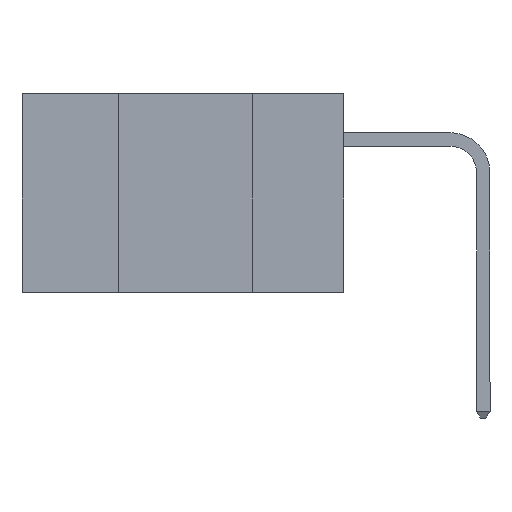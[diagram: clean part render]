
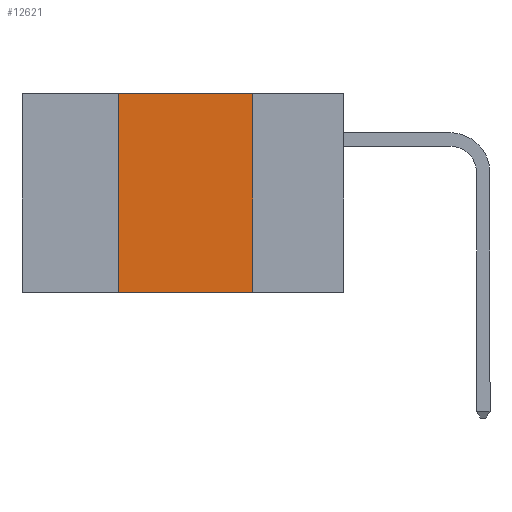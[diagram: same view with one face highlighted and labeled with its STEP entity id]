
A CAD part, left-side view. The second image highlights one B-rep face of the part: STEP entity #12621.
In plain terms, the highlighted planar face has unit normal (-1, 0, 0).
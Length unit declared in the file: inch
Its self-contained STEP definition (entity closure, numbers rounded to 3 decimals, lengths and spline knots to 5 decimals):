
#133 = DIRECTION ( 'NONE',  ( 0., 0., 1. ) ) ;
#1426 = EDGE_CURVE ( 'NONE', #14777, #12174, #7375, .T. ) ;
#1571 = CARTESIAN_POINT ( 'NONE',  ( 0., 0.42, -0.37 ) ) ;
#2990 = VERTEX_POINT ( 'NONE', #11616 ) ;
#3334 = EDGE_CURVE ( 'NONE', #15657, #2990, #10416, .T. ) ;
#4120 = EDGE_LOOP ( 'NONE', ( #12511, #9905, #12928, #5081 ) ) ;
#4126 = VECTOR ( 'NONE', #10595, 39.37008 ) ;
#4680 = DIRECTION ( 'NONE',  ( 0., -1., 0. ) ) ;
#5081 = ORIENTED_EDGE ( 'NONE', *, *, #3334, .T. ) ;
#6603 = VECTOR ( 'NONE', #4680, 39.37008 ) ;
#7154 = VECTOR ( 'NONE', #133, 39.37008 ) ;
#7375 = LINE ( 'NONE', #16394, #17864 ) ;
#7594 = LINE ( 'NONE', #14381, #7154 ) ;
#8070 = PLANE ( 'NONE',  #17657 ) ;
#9606 = DIRECTION ( 'NONE',  ( 0., 0., -1. ) ) ;
#9704 = EDGE_CURVE ( 'NONE', #15657, #14777, #7594, .T. ) ;
#9905 = ORIENTED_EDGE ( 'NONE', *, *, #1426, .F. ) ;
#10416 = LINE ( 'NONE', #12460, #6603 ) ;
#10595 = DIRECTION ( 'NONE',  ( 0., 0., -1. ) ) ;
#11380 = CARTESIAN_POINT ( 'NONE',  ( 0., 0.17, 0. ) ) ;
#11616 = CARTESIAN_POINT ( 'NONE',  ( 0., 0.17, -0.37 ) ) ;
#12032 = CARTESIAN_POINT ( 'NONE',  ( 0., 0.17, 0. ) ) ;
#12174 = VERTEX_POINT ( 'NONE', #11380 ) ;
#12460 = CARTESIAN_POINT ( 'NONE',  ( 0., 0.6, -0.37 ) ) ;
#12499 = CARTESIAN_POINT ( 'NONE',  ( 0., 0.42, 0. ) ) ;
#12511 = ORIENTED_EDGE ( 'NONE', *, *, #13112, .F. ) ;
#12621 = ADVANCED_FACE ( 'NONE', ( #16438 ), #8070, .F. ) ;
#12928 = ORIENTED_EDGE ( 'NONE', *, *, #9704, .F. ) ;
#13112 = EDGE_CURVE ( 'NONE', #12174, #2990, #15531, .T. ) ;
#14381 = CARTESIAN_POINT ( 'NONE',  ( 0., 0.42, 0. ) ) ;
#14777 = VERTEX_POINT ( 'NONE', #12499 ) ;
#15531 = LINE ( 'NONE', #12032, #4126 ) ;
#15657 = VERTEX_POINT ( 'NONE', #1571 ) ;
#16394 = CARTESIAN_POINT ( 'NONE',  ( 0., 0.6, 0. ) ) ;
#16412 = DIRECTION ( 'NONE',  ( 0., -1., 0. ) ) ;
#16438 = FACE_OUTER_BOUND ( 'NONE', #4120, .T. ) ;
#16687 = CARTESIAN_POINT ( 'NONE',  ( 0., 0.6, 0. ) ) ;
#17657 = AXIS2_PLACEMENT_3D ( 'NONE', #16687, #18124, #9606 ) ;
#17864 = VECTOR ( 'NONE', #16412, 39.37008 ) ;
#18124 = DIRECTION ( 'NONE',  ( 1., 0., 0. ) ) ;
